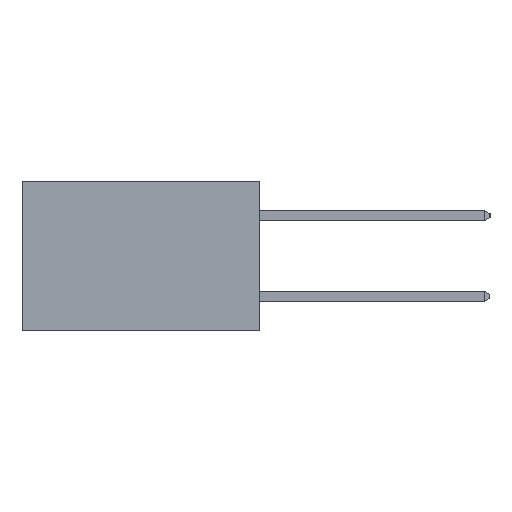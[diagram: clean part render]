
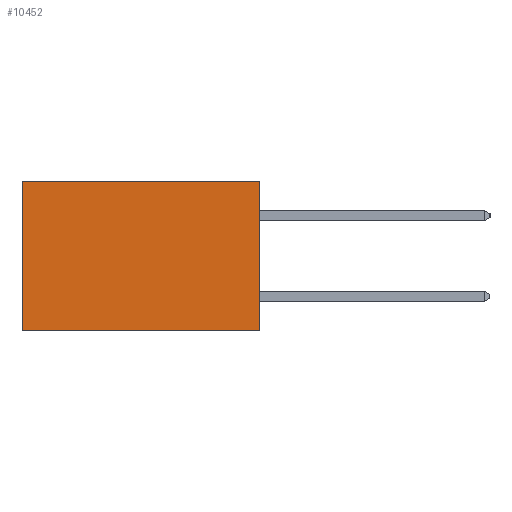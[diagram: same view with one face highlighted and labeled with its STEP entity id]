
A CAD part, left-side view. The second image highlights one B-rep face of the part: STEP entity #10452.
In plain terms, the highlighted planar face has unit normal (-1, 0, 0).
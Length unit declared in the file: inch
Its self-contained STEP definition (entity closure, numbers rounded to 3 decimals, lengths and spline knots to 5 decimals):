
#1679 = CARTESIAN_POINT ( 'NONE',  ( 0.277, 0., 0. ) ) ;
#1906 = VERTEX_POINT ( 'NONE', #7938 ) ;
#2207 = LINE ( 'NONE', #15429, #6630 ) ;
#2426 = VERTEX_POINT ( 'NONE', #8740 ) ;
#2895 = LINE ( 'NONE', #4631, #19168 ) ;
#3507 = CARTESIAN_POINT ( 'NONE',  ( 0.277, 0.59, -0.37 ) ) ;
#3964 = ORIENTED_EDGE ( 'NONE', *, *, #18956, .F. ) ;
#4206 = CARTESIAN_POINT ( 'NONE',  ( 0.277, 0., -0.37 ) ) ;
#4238 = LINE ( 'NONE', #19450, #8103 ) ;
#4631 = CARTESIAN_POINT ( 'NONE',  ( 0.277, 0.59, -0.37 ) ) ;
#5607 = DIRECTION ( 'NONE',  ( 0., 1., 0. ) ) ;
#6574 = DIRECTION ( 'NONE',  ( 1., 0., 0. ) ) ;
#6630 = VECTOR ( 'NONE', #5607, 39.37008 ) ;
#7762 = VERTEX_POINT ( 'NONE', #4206 ) ;
#7938 = CARTESIAN_POINT ( 'NONE',  ( 0.277, 0., 0. ) ) ;
#8103 = VECTOR ( 'NONE', #9841, 39.37008 ) ;
#8242 = LINE ( 'NONE', #1679, #20981 ) ;
#8334 = ORIENTED_EDGE ( 'NONE', *, *, #11127, .F. ) ;
#8740 = CARTESIAN_POINT ( 'NONE',  ( 0.277, 0.59, 0. ) ) ;
#9841 = DIRECTION ( 'NONE',  ( 0., 0., -1. ) ) ;
#10452 = ADVANCED_FACE ( 'NONE', ( #12229 ), #16279, .F. ) ;
#11127 = EDGE_CURVE ( 'NONE', #1906, #7762, #4238, .T. ) ;
#11597 = DIRECTION ( 'NONE',  ( 0., 1., 0. ) ) ;
#12229 = FACE_OUTER_BOUND ( 'NONE', #13866, .T. ) ;
#13866 = EDGE_LOOP ( 'NONE', ( #16486, #3964, #8334, #17009 ) ) ;
#14785 = CARTESIAN_POINT ( 'NONE',  ( 0.277, 0., -0.37 ) ) ;
#15429 = CARTESIAN_POINT ( 'NONE',  ( 0.277, 0., -0.37 ) ) ;
#15533 = EDGE_CURVE ( 'NONE', #2426, #20359, #2895, .T. ) ;
#16067 = DIRECTION ( 'NONE',  ( 0., 0., -1. ) ) ;
#16279 = PLANE ( 'NONE',  #20096 ) ;
#16486 = ORIENTED_EDGE ( 'NONE', *, *, #15533, .T. ) ;
#17009 = ORIENTED_EDGE ( 'NONE', *, *, #19590, .T. ) ;
#17953 = DIRECTION ( 'NONE',  ( 0., 0., -1. ) ) ;
#18956 = EDGE_CURVE ( 'NONE', #7762, #20359, #2207, .T. ) ;
#19168 = VECTOR ( 'NONE', #16067, 39.37008 ) ;
#19450 = CARTESIAN_POINT ( 'NONE',  ( 0.277, 0., -0.37 ) ) ;
#19590 = EDGE_CURVE ( 'NONE', #1906, #2426, #8242, .T. ) ;
#20096 = AXIS2_PLACEMENT_3D ( 'NONE', #14785, #6574, #17953 ) ;
#20359 = VERTEX_POINT ( 'NONE', #3507 ) ;
#20981 = VECTOR ( 'NONE', #11597, 39.37008 ) ;
